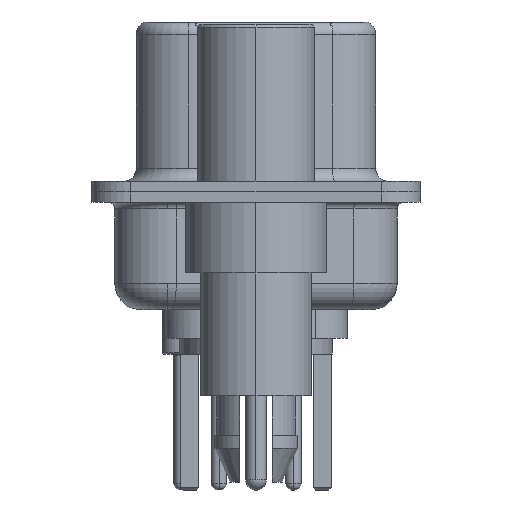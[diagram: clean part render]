
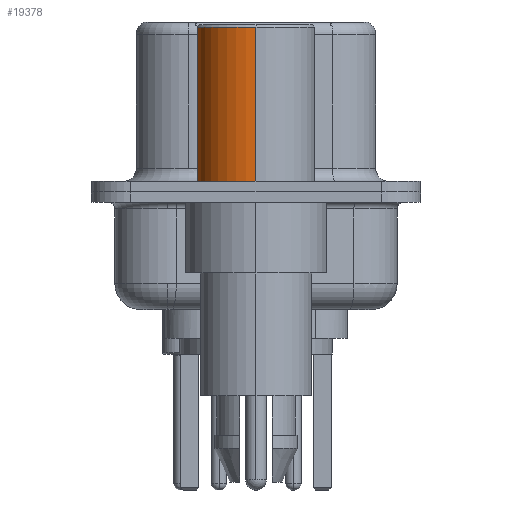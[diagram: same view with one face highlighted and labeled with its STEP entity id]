
A CAD part, left-side view. The second image highlights one B-rep face of the part: STEP entity #19378.
In plain terms, the highlighted cylindrical face has radius 2.25 mm (diameter 4.5 mm), a partial arc.
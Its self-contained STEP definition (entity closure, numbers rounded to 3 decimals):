
#108 = DIRECTION ( 'NONE',  ( 0., 0., 1. ) ) ;
#572 = EDGE_CURVE ( 'NONE', #14066, #17048, #5346, .T. ) ;
#1712 = CYLINDRICAL_SURFACE ( 'NONE', #17219, 2.25 ) ;
#1745 = DIRECTION ( 'NONE',  ( 1., 0., 0. ) ) ;
#1818 = DIRECTION ( 'NONE',  ( 0., 0., 1. ) ) ;
#2173 = ORIENTED_EDGE ( 'NONE', *, *, #19306, .F. ) ;
#2265 = ORIENTED_EDGE ( 'NONE', *, *, #572, .F. ) ;
#2344 = CARTESIAN_POINT ( 'NONE',  ( -2.25, 0., 0.581 ) ) ;
#3687 = CARTESIAN_POINT ( 'NONE',  ( 0., 0., 0.581 ) ) ;
#3967 = CARTESIAN_POINT ( 'NONE',  ( 2.25, 0., 6.3 ) ) ;
#4238 = CARTESIAN_POINT ( 'NONE',  ( -2.25, 0., 6.3 ) ) ;
#4351 = DIRECTION ( 'NONE',  ( 0., 0., 1. ) ) ;
#5346 = LINE ( 'NONE', #16335, #9558 ) ;
#5974 = CARTESIAN_POINT ( 'NONE',  ( -2.25, 0., 0.4 ) ) ;
#6838 = EDGE_CURVE ( 'NONE', #14066, #20825, #10190, .T. ) ;
#8539 = EDGE_CURVE ( 'NONE', #20825, #16015, #18767, .T. ) ;
#8675 = AXIS2_PLACEMENT_3D ( 'NONE', #23330, #12520, #1745 ) ;
#9493 = AXIS2_PLACEMENT_3D ( 'NONE', #15204, #4351, #17032 ) ;
#9558 = VECTOR ( 'NONE', #1818, 1000. ) ;
#9798 = ORIENTED_EDGE ( 'NONE', *, *, #8539, .T. ) ;
#10190 = CIRCLE ( 'NONE', #9493, 2.25 ) ;
#10827 = CARTESIAN_POINT ( 'NONE',  ( 2.25, 0., 0.4 ) ) ;
#11249 = FACE_OUTER_BOUND ( 'NONE', #14565, .T. ) ;
#12520 = DIRECTION ( 'NONE',  ( 0., 0., 1. ) ) ;
#13940 = VECTOR ( 'NONE', #18606, 1000. ) ;
#14066 = VERTEX_POINT ( 'NONE', #10827 ) ;
#14565 = EDGE_LOOP ( 'NONE', ( #16623, #9798, #2173, #2265 ) ) ;
#15204 = CARTESIAN_POINT ( 'NONE',  ( 0., 0., 0.4 ) ) ;
#16015 = VERTEX_POINT ( 'NONE', #4238 ) ;
#16335 = CARTESIAN_POINT ( 'NONE',  ( 2.25, 0., 0.581 ) ) ;
#16339 = DIRECTION ( 'NONE',  ( 1., 0., 0. ) ) ;
#16623 = ORIENTED_EDGE ( 'NONE', *, *, #6838, .T. ) ;
#17032 = DIRECTION ( 'NONE',  ( 1., 0., 0. ) ) ;
#17048 = VERTEX_POINT ( 'NONE', #3967 ) ;
#17219 = AXIS2_PLACEMENT_3D ( 'NONE', #3687, #108, #16339 ) ;
#18606 = DIRECTION ( 'NONE',  ( 0., 0., 1. ) ) ;
#18767 = LINE ( 'NONE', #2344, #13940 ) ;
#19306 = EDGE_CURVE ( 'NONE', #17048, #16015, #22579, .T. ) ;
#19378 = ADVANCED_FACE ( 'NONE', ( #11249 ), #1712, .T. ) ;
#20825 = VERTEX_POINT ( 'NONE', #5974 ) ;
#22579 = CIRCLE ( 'NONE', #8675, 2.25 ) ;
#23330 = CARTESIAN_POINT ( 'NONE',  ( 0., 0., 6.3 ) ) ;
